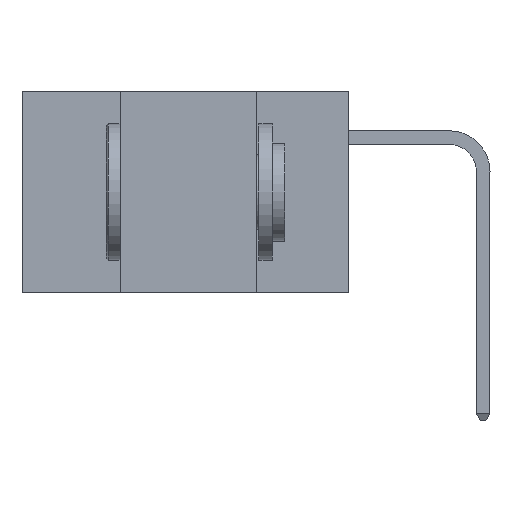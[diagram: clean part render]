
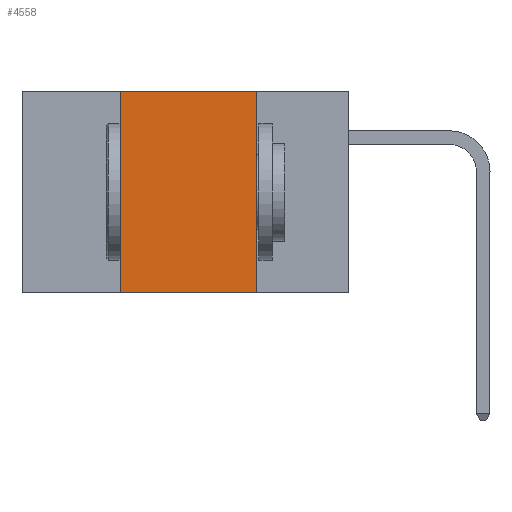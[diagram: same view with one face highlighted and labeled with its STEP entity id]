
A CAD part, left-side view. The second image highlights one B-rep face of the part: STEP entity #4558.
In plain terms, the highlighted planar face has unit normal (-1, 0, 0).
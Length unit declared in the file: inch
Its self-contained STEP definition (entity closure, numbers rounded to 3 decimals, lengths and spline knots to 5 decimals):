
#823 = LINE ( 'NONE', #848, #10867 ) ;
#848 = CARTESIAN_POINT ( 'NONE',  ( 0., 0.6, -0.37 ) ) ;
#862 = DIRECTION ( 'NONE',  ( 0., 0., -1. ) ) ;
#4151 = CARTESIAN_POINT ( 'NONE',  ( 0., 0.17, 0. ) ) ;
#4175 = CARTESIAN_POINT ( 'NONE',  ( 0., 0.17, 0. ) ) ;
#4558 = ADVANCED_FACE ( 'NONE', ( #19220 ), #15992, .F. ) ;
#5552 = DIRECTION ( 'NONE',  ( 0., 0., 1. ) ) ;
#8365 = LINE ( 'NONE', #4151, #39733 ) ;
#10504 = EDGE_CURVE ( 'NONE', #27574, #25396, #16125, .T. ) ;
#10867 = VECTOR ( 'NONE', #32012, 39.37008 ) ;
#13630 = CARTESIAN_POINT ( 'NONE',  ( 0., 0.42, -0.37 ) ) ;
#15252 = VERTEX_POINT ( 'NONE', #15972 ) ;
#15972 = CARTESIAN_POINT ( 'NONE',  ( 0., 0.17, -0.37 ) ) ;
#15992 = PLANE ( 'NONE',  #31293 ) ;
#16125 = LINE ( 'NONE', #25883, #39777 ) ;
#18238 = EDGE_LOOP ( 'NONE', ( #29497, #35052, #39605, #23627 ) ) ;
#18864 = EDGE_CURVE ( 'NONE', #25396, #15252, #8365, .T. ) ;
#19220 = FACE_OUTER_BOUND ( 'NONE', #18238, .T. ) ;
#20025 = VERTEX_POINT ( 'NONE', #13630 ) ;
#23627 = ORIENTED_EDGE ( 'NONE', *, *, #36945, .T. ) ;
#23672 = LINE ( 'NONE', #33293, #38680 ) ;
#25396 = VERTEX_POINT ( 'NONE', #4175 ) ;
#25663 = CARTESIAN_POINT ( 'NONE',  ( 0., 0.6, 0. ) ) ;
#25883 = CARTESIAN_POINT ( 'NONE',  ( 0., 0.6, 0. ) ) ;
#27574 = VERTEX_POINT ( 'NONE', #35773 ) ;
#28387 = DIRECTION ( 'NONE',  ( 1., 0., 0. ) ) ;
#28732 = DIRECTION ( 'NONE',  ( 0., -1., 0. ) ) ;
#29497 = ORIENTED_EDGE ( 'NONE', *, *, #18864, .F. ) ;
#31293 = AXIS2_PLACEMENT_3D ( 'NONE', #25663, #28387, #862 ) ;
#32012 = DIRECTION ( 'NONE',  ( 0., -1., 0. ) ) ;
#33293 = CARTESIAN_POINT ( 'NONE',  ( 0., 0.42, 0. ) ) ;
#34837 = DIRECTION ( 'NONE',  ( 0., 0., -1. ) ) ;
#35052 = ORIENTED_EDGE ( 'NONE', *, *, #10504, .F. ) ;
#35773 = CARTESIAN_POINT ( 'NONE',  ( 0., 0.42, 0. ) ) ;
#36945 = EDGE_CURVE ( 'NONE', #20025, #15252, #823, .T. ) ;
#38680 = VECTOR ( 'NONE', #5552, 39.37008 ) ;
#38700 = EDGE_CURVE ( 'NONE', #20025, #27574, #23672, .T. ) ;
#39605 = ORIENTED_EDGE ( 'NONE', *, *, #38700, .F. ) ;
#39733 = VECTOR ( 'NONE', #34837, 39.37008 ) ;
#39777 = VECTOR ( 'NONE', #28732, 39.37008 ) ;
